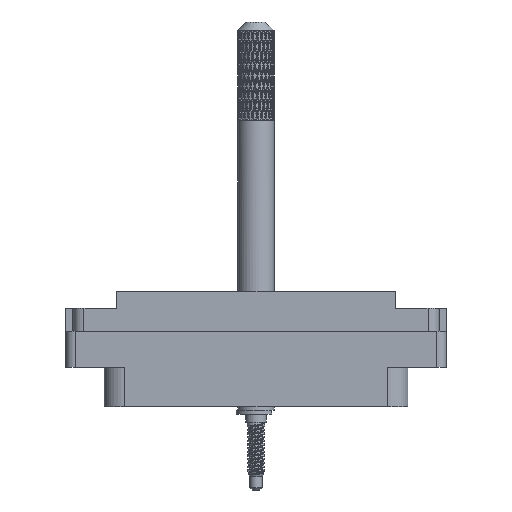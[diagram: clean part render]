
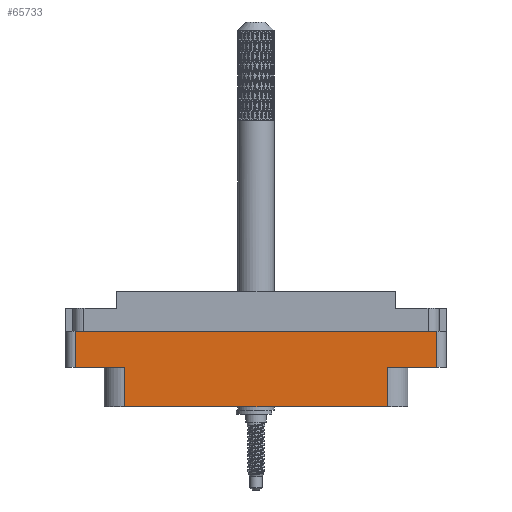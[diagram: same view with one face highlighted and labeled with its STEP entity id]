
A CAD part, front view. The second image highlights one B-rep face of the part: STEP entity #65733.
In plain terms, the highlighted planar face has unit normal (0, -1, 0).
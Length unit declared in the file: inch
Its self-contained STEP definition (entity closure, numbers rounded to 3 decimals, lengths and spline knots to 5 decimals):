
#2345 = VECTOR ( 'NONE', #95981, 39.37008 ) ;
#3687 = DIRECTION ( 'NONE',  ( 0., 0., 1. ) ) ;
#4898 = CARTESIAN_POINT ( 'NONE',  ( 0., -0.438, -0.274 ) ) ;
#5965 = VECTOR ( 'NONE', #37741, 39.37008 ) ;
#6092 = EDGE_CURVE ( 'NONE', #97978, #23332, #98007, .T. ) ;
#7117 = VERTEX_POINT ( 'NONE', #23436 ) ;
#11387 = ORIENTED_EDGE ( 'NONE', *, *, #79609, .T. ) ;
#12694 = CARTESIAN_POINT ( 'NONE',  ( 1.2335, -0.438, -0.52 ) ) ;
#12852 = DIRECTION ( 'NONE',  ( 0., -1., 0. ) ) ;
#13601 = DIRECTION ( 'NONE',  ( 0., 0., -1. ) ) ;
#14925 = VERTEX_POINT ( 'NONE', #12694 ) ;
#16469 = CARTESIAN_POINT ( 'NONE',  ( -1.2335, -0.438, -0.274 ) ) ;
#18998 = VECTOR ( 'NONE', #72899, 39.37008 ) ;
#22792 = DIRECTION ( 'NONE',  ( 0., 0., -1. ) ) ;
#23332 = VERTEX_POINT ( 'NONE', #31570 ) ;
#23436 = CARTESIAN_POINT ( 'NONE',  ( 0.895, -0.438, -0.52 ) ) ;
#25191 = CARTESIAN_POINT ( 'NONE',  ( -1.2335, -0.438, -0.789 ) ) ;
#25353 = EDGE_CURVE ( 'NONE', #14925, #7117, #42436, .T. ) ;
#28407 = VERTEX_POINT ( 'NONE', #16469 ) ;
#28440 = VERTEX_POINT ( 'NONE', #69568 ) ;
#28548 = CARTESIAN_POINT ( 'NONE',  ( 0., -0.438, -0.52 ) ) ;
#29383 = AXIS2_PLACEMENT_3D ( 'NONE', #48083, #12852, #13601 ) ;
#30977 = CARTESIAN_POINT ( 'NONE',  ( -0.895, -0.438, -0.789 ) ) ;
#31353 = EDGE_CURVE ( 'NONE', #97978, #28440, #87809, .T. ) ;
#31570 = CARTESIAN_POINT ( 'NONE',  ( -1.2335, -0.438, -0.52 ) ) ;
#34674 = CARTESIAN_POINT ( 'NONE',  ( -0.895, -0.438, -0.52 ) ) ;
#37741 = DIRECTION ( 'NONE',  ( 1., 0., 0. ) ) ;
#38137 = FACE_OUTER_BOUND ( 'NONE', #108866, .T. ) ;
#42436 = LINE ( 'NONE', #28548, #2345 ) ;
#43099 = CARTESIAN_POINT ( 'NONE',  ( 0.895, -0.438, -0.52 ) ) ;
#44792 = LINE ( 'NONE', #4898, #5965 ) ;
#47691 = PLANE ( 'NONE',  #29383 ) ;
#47975 = ORIENTED_EDGE ( 'NONE', *, *, #100603, .T. ) ;
#48083 = CARTESIAN_POINT ( 'NONE',  ( -1.2955, -0.438, -0.789 ) ) ;
#52552 = VECTOR ( 'NONE', #67862, 39.37008 ) ;
#60397 = VECTOR ( 'NONE', #85178, 39.37008 ) ;
#63864 = CARTESIAN_POINT ( 'NONE',  ( -1.2955, -0.438, -0.789 ) ) ;
#65733 = ADVANCED_FACE ( 'NONE', ( #38137 ), #47691, .T. ) ;
#66530 = VECTOR ( 'NONE', #3687, 39.37008 ) ;
#67862 = DIRECTION ( 'NONE',  ( -1., 0., 0. ) ) ;
#69568 = CARTESIAN_POINT ( 'NONE',  ( -0.895, -0.438, -0.789 ) ) ;
#70486 = DIRECTION ( 'NONE',  ( 0., 0., -1. ) ) ;
#70534 = ORIENTED_EDGE ( 'NONE', *, *, #108148, .F. ) ;
#72899 = DIRECTION ( 'NONE',  ( 1., 0., 0. ) ) ;
#74187 = VECTOR ( 'NONE', #70486, 39.37008 ) ;
#76945 = ORIENTED_EDGE ( 'NONE', *, *, #31353, .T. ) ;
#78393 = VECTOR ( 'NONE', #22792, 39.37008 ) ;
#79609 = EDGE_CURVE ( 'NONE', #88637, #7117, #96598, .T. ) ;
#82453 = ORIENTED_EDGE ( 'NONE', *, *, #25353, .F. ) ;
#84793 = CARTESIAN_POINT ( 'NONE',  ( 0., -0.438, -0.52 ) ) ;
#85178 = DIRECTION ( 'NONE',  ( 0., 0., 1. ) ) ;
#87809 = LINE ( 'NONE', #30977, #78393 ) ;
#88189 = CARTESIAN_POINT ( 'NONE',  ( 1.2335, -0.438, -0.274 ) ) ;
#88637 = VERTEX_POINT ( 'NONE', #102710 ) ;
#88752 = VERTEX_POINT ( 'NONE', #88189 ) ;
#93095 = ORIENTED_EDGE ( 'NONE', *, *, #6092, .F. ) ;
#93616 = EDGE_CURVE ( 'NONE', #28407, #23332, #107605, .T. ) ;
#95981 = DIRECTION ( 'NONE',  ( -1., 0., 0. ) ) ;
#96598 = LINE ( 'NONE', #43099, #60397 ) ;
#97978 = VERTEX_POINT ( 'NONE', #34674 ) ;
#98007 = LINE ( 'NONE', #84793, #52552 ) ;
#98676 = ORIENTED_EDGE ( 'NONE', *, *, #93616, .T. ) ;
#100603 = EDGE_CURVE ( 'NONE', #28440, #88637, #108641, .T. ) ;
#102710 = CARTESIAN_POINT ( 'NONE',  ( 0.895, -0.438, -0.789 ) ) ;
#107245 = CARTESIAN_POINT ( 'NONE',  ( 1.2335, -0.438, -0.789 ) ) ;
#107605 = LINE ( 'NONE', #25191, #74187 ) ;
#107925 = LINE ( 'NONE', #107245, #66530 ) ;
#108148 = EDGE_CURVE ( 'NONE', #28407, #88752, #44792, .T. ) ;
#108641 = LINE ( 'NONE', #63864, #18998 ) ;
#108866 = EDGE_LOOP ( 'NONE', ( #70534, #98676, #93095, #76945, #47975, #11387, #82453, #109503 ) ) ;
#109028 = EDGE_CURVE ( 'NONE', #14925, #88752, #107925, .T. ) ;
#109503 = ORIENTED_EDGE ( 'NONE', *, *, #109028, .T. ) ;
